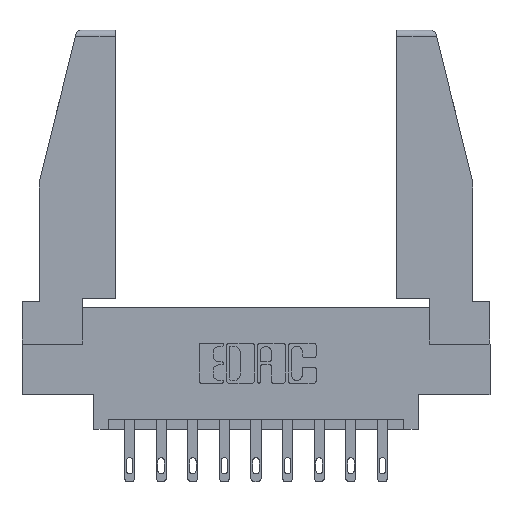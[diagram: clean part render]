
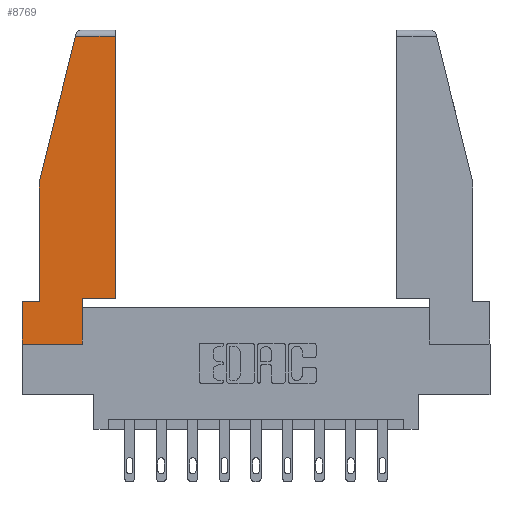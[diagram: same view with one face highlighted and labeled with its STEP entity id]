
A CAD part, top view. The second image highlights one B-rep face of the part: STEP entity #8769.
In plain terms, the highlighted planar face has unit normal (0, 0, 1).
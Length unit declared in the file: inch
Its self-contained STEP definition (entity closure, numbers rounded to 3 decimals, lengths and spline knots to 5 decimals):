
#38 = ORIENTED_EDGE ( 'NONE', *, *, #10156, .T. ) ;
#192 = VERTEX_POINT ( 'NONE', #3443 ) ;
#588 = ORIENTED_EDGE ( 'NONE', *, *, #6549, .T. ) ;
#589 = VERTEX_POINT ( 'NONE', #1927 ) ;
#599 = LINE ( 'NONE', #10330, #5948 ) ;
#701 = EDGE_CURVE ( 'NONE', #12016, #8400, #9011, .T. ) ;
#1269 = CARTESIAN_POINT ( 'NONE',  ( 0.086, 0.8, 0. ) ) ;
#1411 = ORIENTED_EDGE ( 'NONE', *, *, #10367, .T. ) ;
#1421 = PLANE ( 'NONE',  #10903 ) ;
#1486 = DIRECTION ( 'NONE',  ( -0.239, -0.971, 0. ) ) ;
#1667 = LINE ( 'NONE', #4451, #8003 ) ;
#1713 = CARTESIAN_POINT ( 'NONE',  ( 0., 1.52, 0. ) ) ;
#1779 = LINE ( 'NONE', #3551, #9414 ) ;
#1880 = EDGE_CURVE ( 'NONE', #589, #9582, #1667, .T. ) ;
#1927 = CARTESIAN_POINT ( 'NONE',  ( 0.2636, 1.52, 0. ) ) ;
#2263 = ORIENTED_EDGE ( 'NONE', *, *, #1880, .T. ) ;
#2488 = LINE ( 'NONE', #10029, #11754 ) ;
#2752 = ORIENTED_EDGE ( 'NONE', *, *, #701, .T. ) ;
#2909 = CARTESIAN_POINT ( 'NONE',  ( 0., 0., 0. ) ) ;
#3278 = DIRECTION ( 'NONE',  ( -1., 0., 0. ) ) ;
#3443 = CARTESIAN_POINT ( 'NONE',  ( 0., 0., 0. ) ) ;
#3488 = DIRECTION ( 'NONE',  ( 0., -1., 0. ) ) ;
#3551 = CARTESIAN_POINT ( 'NONE',  ( 0., 0.21, 0. ) ) ;
#3959 = CARTESIAN_POINT ( 'NONE',  ( 0.461, 1.52, 0. ) ) ;
#4081 = DIRECTION ( 'NONE',  ( 1., 0., 0. ) ) ;
#4220 = CARTESIAN_POINT ( 'NONE',  ( 0.461, 0.223, 0. ) ) ;
#4451 = CARTESIAN_POINT ( 'NONE',  ( 0.271, 1.55, 0. ) ) ;
#4474 = VECTOR ( 'NONE', #3488, 39.37008 ) ;
#4494 = DIRECTION ( 'NONE',  ( 1., 0., 0. ) ) ;
#4866 = LINE ( 'NONE', #5213, #8355 ) ;
#5213 = CARTESIAN_POINT ( 'NONE',  ( 0., 0., 0. ) ) ;
#5515 = LINE ( 'NONE', #8567, #5677 ) ;
#5677 = VECTOR ( 'NONE', #3278, 39.37008 ) ;
#5948 = VECTOR ( 'NONE', #4081, 39.37008 ) ;
#5974 = DIRECTION ( 'NONE',  ( 0., 0., 1. ) ) ;
#6201 = VECTOR ( 'NONE', #10651, 39.37008 ) ;
#6366 = EDGE_CURVE ( 'NONE', #192, #7055, #4866, .T. ) ;
#6373 = EDGE_LOOP ( 'NONE', ( #2752, #588, #2263, #38, #8801, #7752, #9137, #10858, #1411 ) ) ;
#6549 = EDGE_CURVE ( 'NONE', #8400, #589, #9481, .T. ) ;
#6918 = DIRECTION ( 'NONE',  ( -1., 0., 0. ) ) ;
#7055 = VERTEX_POINT ( 'NONE', #9750 ) ;
#7550 = CARTESIAN_POINT ( 'NONE',  ( 0.461, 0.223, 0. ) ) ;
#7752 = ORIENTED_EDGE ( 'NONE', *, *, #13468, .T. ) ;
#8003 = VECTOR ( 'NONE', #1486, 39.37008 ) ;
#8355 = VECTOR ( 'NONE', #10530, 39.37008 ) ;
#8400 = VERTEX_POINT ( 'NONE', #3959 ) ;
#8550 = CARTESIAN_POINT ( 'NONE',  ( 0., 0.21, 0. ) ) ;
#8567 = CARTESIAN_POINT ( 'NONE',  ( 0., 0.21, 0. ) ) ;
#8769 = ADVANCED_FACE ( 'NONE', ( #12941 ), #1421, .T. ) ;
#8801 = ORIENTED_EDGE ( 'NONE', *, *, #12061, .T. ) ;
#9011 = LINE ( 'NONE', #4220, #6201 ) ;
#9057 = VERTEX_POINT ( 'NONE', #11021 ) ;
#9137 = ORIENTED_EDGE ( 'NONE', *, *, #6366, .T. ) ;
#9377 = VERTEX_POINT ( 'NONE', #12492 ) ;
#9414 = VECTOR ( 'NONE', #11976, 39.37008 ) ;
#9481 = LINE ( 'NONE', #1713, #11481 ) ;
#9582 = VERTEX_POINT ( 'NONE', #12338 ) ;
#9738 = VERTEX_POINT ( 'NONE', #8550 ) ;
#9750 = CARTESIAN_POINT ( 'NONE',  ( 0.297, 0., 0. ) ) ;
#10029 = CARTESIAN_POINT ( 'NONE',  ( 0.297, 0., 0. ) ) ;
#10156 = EDGE_CURVE ( 'NONE', #9582, #9377, #13752, .T. ) ;
#10330 = CARTESIAN_POINT ( 'NONE',  ( 0.297, 0.223, 0. ) ) ;
#10367 = EDGE_CURVE ( 'NONE', #9057, #12016, #599, .T. ) ;
#10530 = DIRECTION ( 'NONE',  ( 1., 0., 0. ) ) ;
#10651 = DIRECTION ( 'NONE',  ( 0., 1., 0. ) ) ;
#10858 = ORIENTED_EDGE ( 'NONE', *, *, #13182, .T. ) ;
#10903 = AXIS2_PLACEMENT_3D ( 'NONE', #2909, #5974, #4494 ) ;
#11021 = CARTESIAN_POINT ( 'NONE',  ( 0.297, 0.223, 0. ) ) ;
#11096 = DIRECTION ( 'NONE',  ( 0., 1., 0. ) ) ;
#11481 = VECTOR ( 'NONE', #6918, 39.37008 ) ;
#11754 = VECTOR ( 'NONE', #11096, 39.37008 ) ;
#11976 = DIRECTION ( 'NONE',  ( 0., -1., 0. ) ) ;
#12016 = VERTEX_POINT ( 'NONE', #7550 ) ;
#12061 = EDGE_CURVE ( 'NONE', #9377, #9738, #5515, .T. ) ;
#12338 = CARTESIAN_POINT ( 'NONE',  ( 0.086, 0.8, 0. ) ) ;
#12492 = CARTESIAN_POINT ( 'NONE',  ( 0.086, 0.21, 0. ) ) ;
#12941 = FACE_OUTER_BOUND ( 'NONE', #6373, .T. ) ;
#13182 = EDGE_CURVE ( 'NONE', #7055, #9057, #2488, .T. ) ;
#13468 = EDGE_CURVE ( 'NONE', #9738, #192, #1779, .T. ) ;
#13752 = LINE ( 'NONE', #1269, #4474 ) ;
